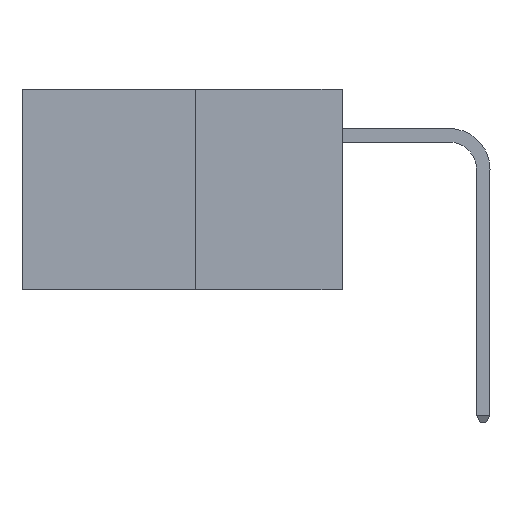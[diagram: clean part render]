
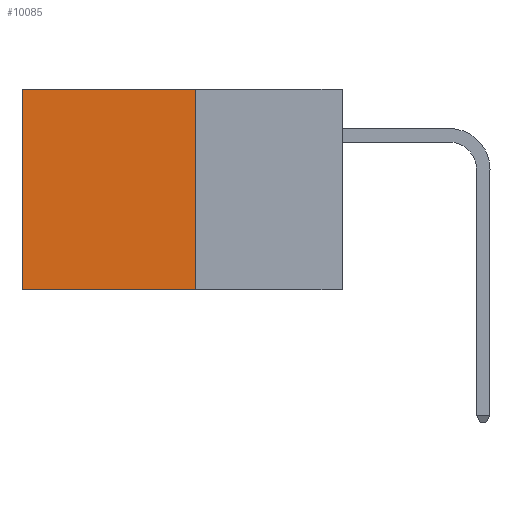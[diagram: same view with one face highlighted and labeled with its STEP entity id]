
A CAD part, left-side view. The second image highlights one B-rep face of the part: STEP entity #10085.
In plain terms, the highlighted planar face has unit normal (-1, 0, 0).
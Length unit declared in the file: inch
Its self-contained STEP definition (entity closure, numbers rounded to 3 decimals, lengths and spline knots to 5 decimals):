
#116 = VERTEX_POINT ( 'NONE', #8046 ) ;
#396 = ORIENTED_EDGE ( 'NONE', *, *, #5200, .T. ) ;
#499 = CARTESIAN_POINT ( 'NONE',  ( 0.277, 0.59, -0.37 ) ) ;
#577 = FACE_OUTER_BOUND ( 'NONE', #4002, .T. ) ;
#591 = CARTESIAN_POINT ( 'NONE',  ( 0.277, 0.27, -0.37 ) ) ;
#994 = VECTOR ( 'NONE', #8900, 39.37008 ) ;
#1037 = VERTEX_POINT ( 'NONE', #4546 ) ;
#1316 = LINE ( 'NONE', #499, #994 ) ;
#1636 = DIRECTION ( 'NONE',  ( 0., 0., -1. ) ) ;
#2140 = LINE ( 'NONE', #11167, #9408 ) ;
#2229 = CARTESIAN_POINT ( 'NONE',  ( 0.277, 0.27, 0. ) ) ;
#2315 = LINE ( 'NONE', #7416, #11055 ) ;
#3366 = EDGE_CURVE ( 'NONE', #6226, #1037, #2315, .T. ) ;
#4002 = EDGE_LOOP ( 'NONE', ( #7475, #7280, #6919, #396 ) ) ;
#4312 = EDGE_CURVE ( 'NONE', #9950, #116, #1316, .T. ) ;
#4546 = CARTESIAN_POINT ( 'NONE',  ( 0.277, 0.27, -0.37 ) ) ;
#4729 = CARTESIAN_POINT ( 'NONE',  ( 0.277, 0.27, 0. ) ) ;
#5200 = EDGE_CURVE ( 'NONE', #6226, #9950, #11527, .T. ) ;
#5406 = PLANE ( 'NONE',  #7053 ) ;
#5956 = DIRECTION ( 'NONE',  ( 0., 1., 0. ) ) ;
#6226 = VERTEX_POINT ( 'NONE', #4729 ) ;
#6601 = VECTOR ( 'NONE', #9501, 39.37008 ) ;
#6919 = ORIENTED_EDGE ( 'NONE', *, *, #3366, .F. ) ;
#6972 = CARTESIAN_POINT ( 'NONE',  ( 0.277, 0.59, 0. ) ) ;
#7053 = AXIS2_PLACEMENT_3D ( 'NONE', #591, #7200, #1636 ) ;
#7200 = DIRECTION ( 'NONE',  ( 1., 0., 0. ) ) ;
#7280 = ORIENTED_EDGE ( 'NONE', *, *, #11749, .F. ) ;
#7416 = CARTESIAN_POINT ( 'NONE',  ( 0.277, 0.27, -0.37 ) ) ;
#7475 = ORIENTED_EDGE ( 'NONE', *, *, #4312, .T. ) ;
#8046 = CARTESIAN_POINT ( 'NONE',  ( 0.277, 0.59, -0.37 ) ) ;
#8900 = DIRECTION ( 'NONE',  ( 0., 0., -1. ) ) ;
#9408 = VECTOR ( 'NONE', #5956, 39.37008 ) ;
#9501 = DIRECTION ( 'NONE',  ( 0., 1., 0. ) ) ;
#9950 = VERTEX_POINT ( 'NONE', #6972 ) ;
#10085 = ADVANCED_FACE ( 'NONE', ( #577 ), #5406, .F. ) ;
#10470 = DIRECTION ( 'NONE',  ( 0., 0., -1. ) ) ;
#11055 = VECTOR ( 'NONE', #10470, 39.37008 ) ;
#11167 = CARTESIAN_POINT ( 'NONE',  ( 0.277, 0.27, -0.37 ) ) ;
#11527 = LINE ( 'NONE', #2229, #6601 ) ;
#11749 = EDGE_CURVE ( 'NONE', #1037, #116, #2140, .T. ) ;
